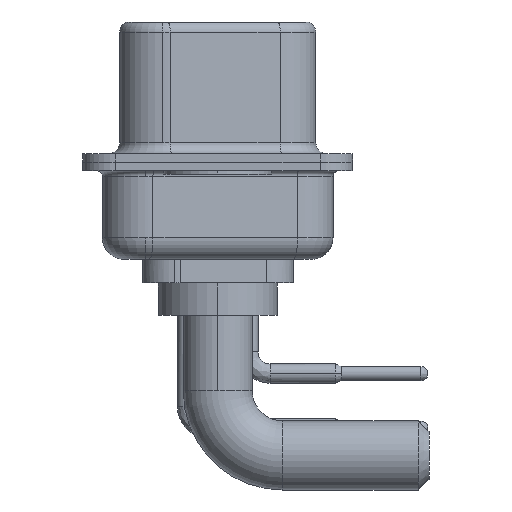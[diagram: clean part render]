
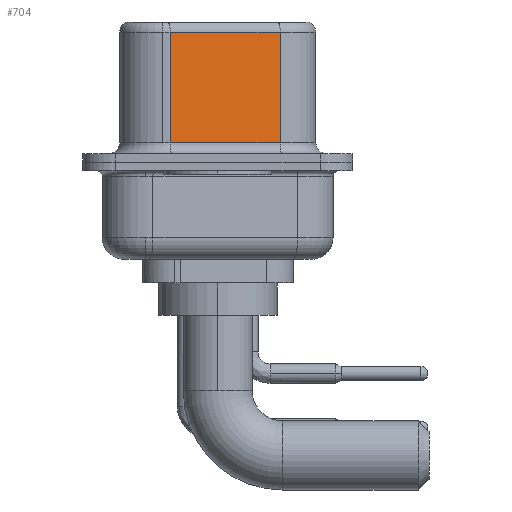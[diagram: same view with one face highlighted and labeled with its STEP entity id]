
A CAD part, left-side view. The second image highlights one B-rep face of the part: STEP entity #704.
In plain terms, the highlighted planar face has unit normal (-0.985, -0.174, 0).
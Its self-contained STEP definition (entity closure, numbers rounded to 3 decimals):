
#28 = EDGE_CURVE ( 'NONE', #10460, #3579, #15878, .T. ) ;
#704 = ADVANCED_FACE ( 'NONE', ( #15089 ), #783, .F. ) ;
#783 = PLANE ( 'NONE',  #1218 ) ;
#885 = DIRECTION ( 'NONE',  ( -0.174, 0.985, 0. ) ) ;
#1218 = AXIS2_PLACEMENT_3D ( 'NONE', #10274, #8808, #885 ) ;
#1804 = CARTESIAN_POINT ( 'NONE',  ( 3.68, 2.203, 6.02 ) ) ;
#1927 = LINE ( 'NONE', #5152, #9907 ) ;
#2229 = ORIENTED_EDGE ( 'NONE', *, *, #18969, .T. ) ;
#2783 = ORIENTED_EDGE ( 'NONE', *, *, #7647, .T. ) ;
#3579 = VERTEX_POINT ( 'NONE', #11439 ) ;
#4063 = EDGE_CURVE ( 'NONE', #5912, #3579, #1927, .T. ) ;
#4488 = VERTEX_POINT ( 'NONE', #1804 ) ;
#5152 = CARTESIAN_POINT ( 'NONE',  ( 4.58, -2.897, 6.52 ) ) ;
#5912 = VERTEX_POINT ( 'NONE', #13596 ) ;
#6074 = VECTOR ( 'NONE', #19418, 1000. ) ;
#6174 = DIRECTION ( 'NONE',  ( 0.174, -0.985, 0. ) ) ;
#7647 = EDGE_CURVE ( 'NONE', #5912, #4488, #17215, .T. ) ;
#7926 = CARTESIAN_POINT ( 'NONE',  ( 4.58, -2.897, 0.9 ) ) ;
#8408 = ORIENTED_EDGE ( 'NONE', *, *, #4063, .F. ) ;
#8808 = DIRECTION ( 'NONE',  ( 0.985, 0.174, 0. ) ) ;
#9175 = DIRECTION ( 'NONE',  ( -0.174, 0.985, 0. ) ) ;
#9907 = VECTOR ( 'NONE', #14454, 1000. ) ;
#10274 = CARTESIAN_POINT ( 'NONE',  ( 4.58, -2.897, 6.52 ) ) ;
#10460 = VERTEX_POINT ( 'NONE', #18862 ) ;
#10709 = ORIENTED_EDGE ( 'NONE', *, *, #28, .T. ) ;
#11439 = CARTESIAN_POINT ( 'NONE',  ( 4.58, -2.897, 0.9 ) ) ;
#11677 = EDGE_LOOP ( 'NONE', ( #8408, #2783, #2229, #10709 ) ) ;
#13596 = CARTESIAN_POINT ( 'NONE',  ( 4.58, -2.897, 6.02 ) ) ;
#14454 = DIRECTION ( 'NONE',  ( 0., 0., -1. ) ) ;
#15089 = FACE_OUTER_BOUND ( 'NONE', #11677, .T. ) ;
#15309 = VECTOR ( 'NONE', #6174, 1000. ) ;
#15878 = LINE ( 'NONE', #7926, #15309 ) ;
#15989 = VECTOR ( 'NONE', #9175, 1000. ) ;
#16186 = CARTESIAN_POINT ( 'NONE',  ( 3.68, 2.203, 6.52 ) ) ;
#17215 = LINE ( 'NONE', #20348, #15989 ) ;
#18862 = CARTESIAN_POINT ( 'NONE',  ( 3.68, 2.203, 0.9 ) ) ;
#18969 = EDGE_CURVE ( 'NONE', #4488, #10460, #19515, .T. ) ;
#19418 = DIRECTION ( 'NONE',  ( 0., 0., -1. ) ) ;
#19515 = LINE ( 'NONE', #16186, #6074 ) ;
#20348 = CARTESIAN_POINT ( 'NONE',  ( 4.58, -2.897, 6.02 ) ) ;
